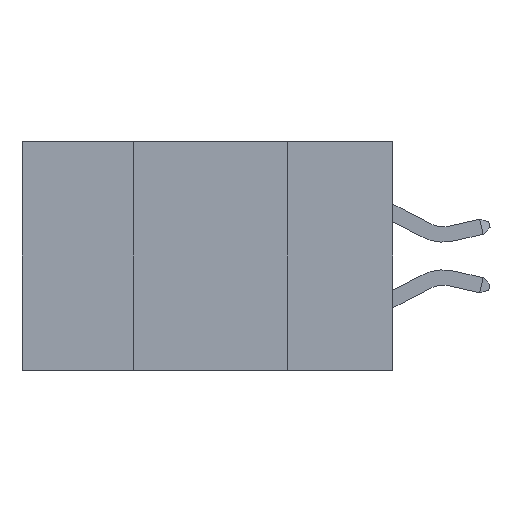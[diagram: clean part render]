
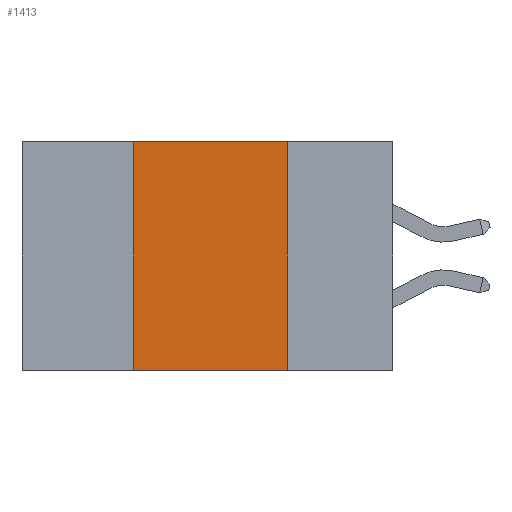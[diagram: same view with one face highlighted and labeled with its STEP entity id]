
A CAD part, left-side view. The second image highlights one B-rep face of the part: STEP entity #1413.
In plain terms, the highlighted planar face has unit normal (-1, 0, 0).
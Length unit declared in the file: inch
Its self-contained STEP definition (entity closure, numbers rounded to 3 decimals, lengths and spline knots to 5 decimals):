
#278 = EDGE_CURVE ( 'NONE', #2373, #1712, #5916, .T. ) ;
#1288 = CARTESIAN_POINT ( 'NONE',  ( 0., 0.17, -0.37 ) ) ;
#1413 = ADVANCED_FACE ( 'NONE', ( #9242 ), #8227, .F. ) ;
#1712 = VERTEX_POINT ( 'NONE', #1835 ) ;
#1835 = CARTESIAN_POINT ( 'NONE',  ( 0., 0.17, 0. ) ) ;
#1910 = VERTEX_POINT ( 'NONE', #7676 ) ;
#2215 = AXIS2_PLACEMENT_3D ( 'NONE', #5599, #7283, #7273 ) ;
#2373 = VERTEX_POINT ( 'NONE', #7132 ) ;
#2546 = EDGE_LOOP ( 'NONE', ( #8175, #8562, #8955, #8950 ) ) ;
#2549 = VECTOR ( 'NONE', #3650, 39.37008 ) ;
#2687 = VERTEX_POINT ( 'NONE', #1288 ) ;
#3566 = CARTESIAN_POINT ( 'NONE',  ( 0., 0.6, 0. ) ) ;
#3622 = VECTOR ( 'NONE', #6569, 39.37008 ) ;
#3650 = DIRECTION ( 'NONE',  ( 0., 0., -1. ) ) ;
#3887 = VECTOR ( 'NONE', #5617, 39.37008 ) ;
#4336 = EDGE_CURVE ( 'NONE', #1910, #2687, #9769, .T. ) ;
#4423 = VECTOR ( 'NONE', #9137, 39.37008 ) ;
#4678 = EDGE_CURVE ( 'NONE', #1910, #2373, #9088, .T. ) ;
#5599 = CARTESIAN_POINT ( 'NONE',  ( 0., 0.6, 0. ) ) ;
#5617 = DIRECTION ( 'NONE',  ( 0., -1., 0. ) ) ;
#5699 = EDGE_CURVE ( 'NONE', #1712, #2687, #6428, .T. ) ;
#5916 = LINE ( 'NONE', #3566, #3887 ) ;
#6328 = CARTESIAN_POINT ( 'NONE',  ( 0., 0.42, 0. ) ) ;
#6428 = LINE ( 'NONE', #7793, #2549 ) ;
#6569 = DIRECTION ( 'NONE',  ( 0., 0., 1. ) ) ;
#7132 = CARTESIAN_POINT ( 'NONE',  ( 0., 0.42, 0. ) ) ;
#7273 = DIRECTION ( 'NONE',  ( 0., 0., -1. ) ) ;
#7283 = DIRECTION ( 'NONE',  ( 1., 0., 0. ) ) ;
#7676 = CARTESIAN_POINT ( 'NONE',  ( 0., 0.42, -0.37 ) ) ;
#7793 = CARTESIAN_POINT ( 'NONE',  ( 0., 0.17, 0. ) ) ;
#8175 = ORIENTED_EDGE ( 'NONE', *, *, #5699, .F. ) ;
#8227 = PLANE ( 'NONE',  #2215 ) ;
#8562 = ORIENTED_EDGE ( 'NONE', *, *, #278, .F. ) ;
#8950 = ORIENTED_EDGE ( 'NONE', *, *, #4336, .T. ) ;
#8955 = ORIENTED_EDGE ( 'NONE', *, *, #4678, .F. ) ;
#9088 = LINE ( 'NONE', #6328, #3622 ) ;
#9137 = DIRECTION ( 'NONE',  ( 0., -1., 0. ) ) ;
#9193 = CARTESIAN_POINT ( 'NONE',  ( 0., 0.6, -0.37 ) ) ;
#9242 = FACE_OUTER_BOUND ( 'NONE', #2546, .T. ) ;
#9769 = LINE ( 'NONE', #9193, #4423 ) ;
